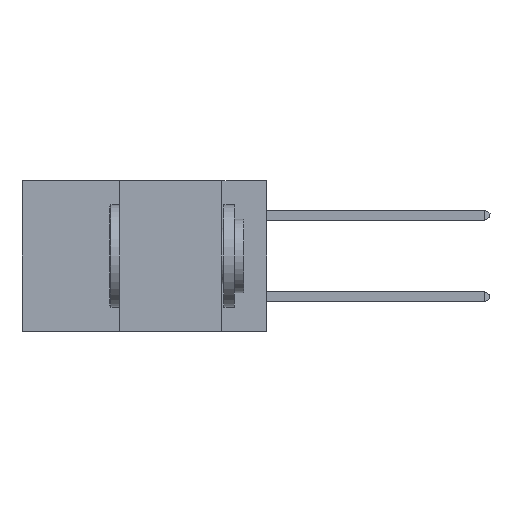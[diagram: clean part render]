
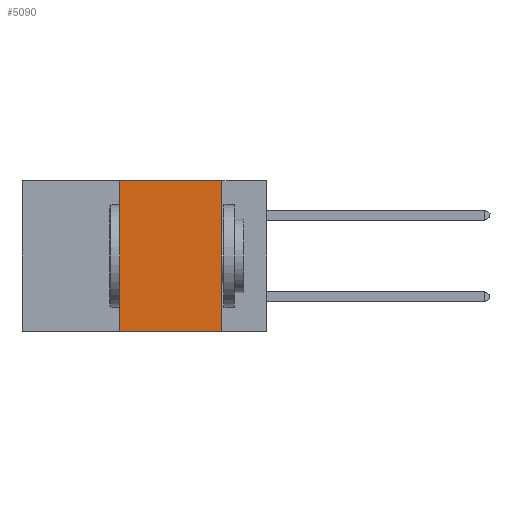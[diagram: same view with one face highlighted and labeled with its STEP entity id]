
A CAD part, left-side view. The second image highlights one B-rep face of the part: STEP entity #5090.
In plain terms, the highlighted planar face has unit normal (-1, 0, 0).
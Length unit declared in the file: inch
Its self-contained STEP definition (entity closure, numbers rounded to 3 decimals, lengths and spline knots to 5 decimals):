
#417 = AXIS2_PLACEMENT_3D ( 'NONE', #2563, #8188, #3352 ) ;
#452 = LINE ( 'NONE', #6222, #6828 ) ;
#473 = CARTESIAN_POINT ( 'NONE',  ( 0., 0.11, 0. ) ) ;
#502 = VERTEX_POINT ( 'NONE', #8165 ) ;
#667 = EDGE_CURVE ( 'NONE', #4350, #8919, #5489, .T. ) ;
#822 = PLANE ( 'NONE',  #417 ) ;
#1696 = EDGE_LOOP ( 'NONE', ( #4802, #5764, #4216, #5152 ) ) ;
#2312 = LINE ( 'NONE', #4988, #3960 ) ;
#2563 = CARTESIAN_POINT ( 'NONE',  ( 0., 0.6, 0. ) ) ;
#2600 = EDGE_CURVE ( 'NONE', #4431, #8919, #2960, .T. ) ;
#2700 = CARTESIAN_POINT ( 'NONE',  ( 0., 0.36, -0.37 ) ) ;
#2929 = DIRECTION ( 'NONE',  ( 0., -1., 0. ) ) ;
#2960 = LINE ( 'NONE', #3087, #6815 ) ;
#3087 = CARTESIAN_POINT ( 'NONE',  ( 0., 0.6, -0.37 ) ) ;
#3352 = DIRECTION ( 'NONE',  ( 0., 0., -1. ) ) ;
#3960 = VECTOR ( 'NONE', #4136, 39.37008 ) ;
#4136 = DIRECTION ( 'NONE',  ( 0., 0., 1. ) ) ;
#4216 = ORIENTED_EDGE ( 'NONE', *, *, #10143, .F. ) ;
#4350 = VERTEX_POINT ( 'NONE', #4472 ) ;
#4431 = VERTEX_POINT ( 'NONE', #2700 ) ;
#4472 = CARTESIAN_POINT ( 'NONE',  ( 0., 0.11, 0. ) ) ;
#4802 = ORIENTED_EDGE ( 'NONE', *, *, #667, .F. ) ;
#4934 = VECTOR ( 'NONE', #7812, 39.37008 ) ;
#4988 = CARTESIAN_POINT ( 'NONE',  ( 0., 0.36, 0. ) ) ;
#5090 = ADVANCED_FACE ( 'NONE', ( #6632 ), #822, .F. ) ;
#5152 = ORIENTED_EDGE ( 'NONE', *, *, #2600, .T. ) ;
#5489 = LINE ( 'NONE', #473, #4934 ) ;
#5764 = ORIENTED_EDGE ( 'NONE', *, *, #8192, .F. ) ;
#6222 = CARTESIAN_POINT ( 'NONE',  ( 0., 0.6, 0. ) ) ;
#6632 = FACE_OUTER_BOUND ( 'NONE', #1696, .T. ) ;
#6815 = VECTOR ( 'NONE', #2929, 39.37008 ) ;
#6828 = VECTOR ( 'NONE', #9260, 39.37008 ) ;
#7812 = DIRECTION ( 'NONE',  ( 0., 0., -1. ) ) ;
#8165 = CARTESIAN_POINT ( 'NONE',  ( 0., 0.36, 0. ) ) ;
#8188 = DIRECTION ( 'NONE',  ( 1., 0., 0. ) ) ;
#8192 = EDGE_CURVE ( 'NONE', #502, #4350, #452, .T. ) ;
#8919 = VERTEX_POINT ( 'NONE', #9282 ) ;
#9260 = DIRECTION ( 'NONE',  ( 0., -1., 0. ) ) ;
#9282 = CARTESIAN_POINT ( 'NONE',  ( 0., 0.11, -0.37 ) ) ;
#10143 = EDGE_CURVE ( 'NONE', #4431, #502, #2312, .T. ) ;
